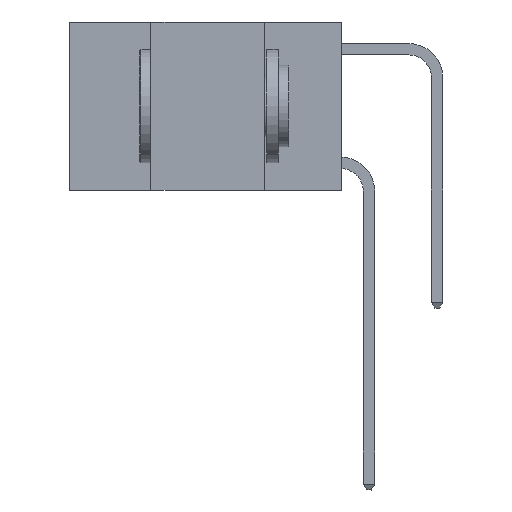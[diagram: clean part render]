
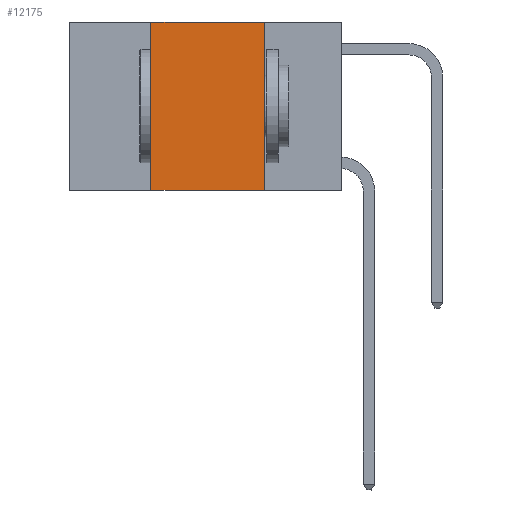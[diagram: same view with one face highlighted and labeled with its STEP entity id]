
A CAD part, left-side view. The second image highlights one B-rep face of the part: STEP entity #12175.
In plain terms, the highlighted planar face has unit normal (-1, 0, 0).
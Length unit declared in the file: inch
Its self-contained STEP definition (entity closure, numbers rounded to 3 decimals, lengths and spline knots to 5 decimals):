
#53 = CARTESIAN_POINT ( 'NONE',  ( 0., 0.6, 0. ) ) ;
#317 = ORIENTED_EDGE ( 'NONE', *, *, #7023, .F. ) ;
#625 = LINE ( 'NONE', #12195, #5529 ) ;
#682 = EDGE_CURVE ( 'NONE', #7556, #947, #9371, .T. ) ;
#947 = VERTEX_POINT ( 'NONE', #5858 ) ;
#1081 = DIRECTION ( 'NONE',  ( 0., -1., 0. ) ) ;
#1183 = CARTESIAN_POINT ( 'NONE',  ( 0., 0.17, 0. ) ) ;
#1468 = CARTESIAN_POINT ( 'NONE',  ( 0., 0.42, -0.37 ) ) ;
#1637 = VERTEX_POINT ( 'NONE', #4097 ) ;
#2368 = DIRECTION ( 'NONE',  ( 0., 0., 1. ) ) ;
#2667 = VECTOR ( 'NONE', #10882, 39.37008 ) ;
#3122 = EDGE_CURVE ( 'NONE', #10313, #1637, #625, .T. ) ;
#3304 = ORIENTED_EDGE ( 'NONE', *, *, #7071, .T. ) ;
#3325 = VECTOR ( 'NONE', #1081, 39.37008 ) ;
#4071 = DIRECTION ( 'NONE',  ( 1., 0., 0. ) ) ;
#4097 = CARTESIAN_POINT ( 'NONE',  ( 0., 0.42, 0. ) ) ;
#4112 = FACE_OUTER_BOUND ( 'NONE', #4815, .T. ) ;
#4233 = LINE ( 'NONE', #12900, #3325 ) ;
#4513 = VECTOR ( 'NONE', #11197, 39.37008 ) ;
#4815 = EDGE_LOOP ( 'NONE', ( #5704, #317, #11600, #3304 ) ) ;
#5529 = VECTOR ( 'NONE', #2368, 39.37008 ) ;
#5704 = ORIENTED_EDGE ( 'NONE', *, *, #682, .F. ) ;
#5746 = PLANE ( 'NONE',  #6813 ) ;
#5858 = CARTESIAN_POINT ( 'NONE',  ( 0., 0.17, -0.37 ) ) ;
#6813 = AXIS2_PLACEMENT_3D ( 'NONE', #53, #4071, #7984 ) ;
#7023 = EDGE_CURVE ( 'NONE', #1637, #7556, #9075, .T. ) ;
#7071 = EDGE_CURVE ( 'NONE', #10313, #947, #4233, .T. ) ;
#7556 = VERTEX_POINT ( 'NONE', #9737 ) ;
#7984 = DIRECTION ( 'NONE',  ( 0., 0., -1. ) ) ;
#9075 = LINE ( 'NONE', #11847, #2667 ) ;
#9371 = LINE ( 'NONE', #1183, #4513 ) ;
#9737 = CARTESIAN_POINT ( 'NONE',  ( 0., 0.17, 0. ) ) ;
#10313 = VERTEX_POINT ( 'NONE', #1468 ) ;
#10882 = DIRECTION ( 'NONE',  ( 0., -1., 0. ) ) ;
#11197 = DIRECTION ( 'NONE',  ( 0., 0., -1. ) ) ;
#11600 = ORIENTED_EDGE ( 'NONE', *, *, #3122, .F. ) ;
#11847 = CARTESIAN_POINT ( 'NONE',  ( 0., 0.6, 0. ) ) ;
#12175 = ADVANCED_FACE ( 'NONE', ( #4112 ), #5746, .F. ) ;
#12195 = CARTESIAN_POINT ( 'NONE',  ( 0., 0.42, 0. ) ) ;
#12900 = CARTESIAN_POINT ( 'NONE',  ( 0., 0.6, -0.37 ) ) ;
